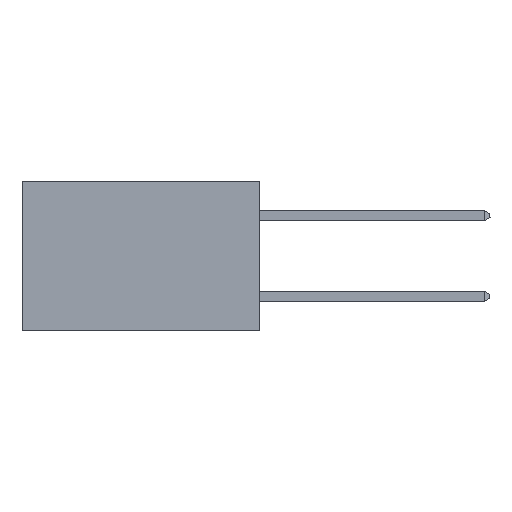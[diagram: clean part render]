
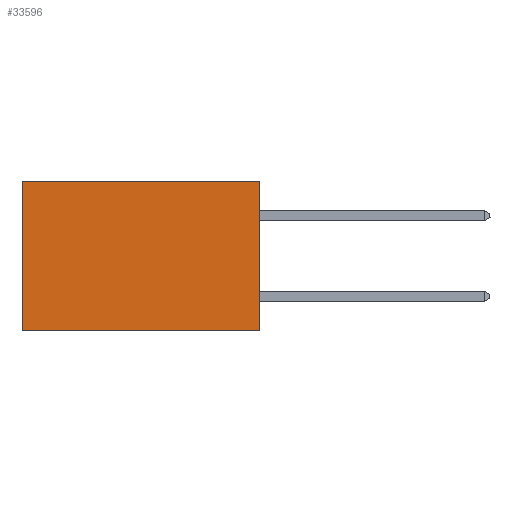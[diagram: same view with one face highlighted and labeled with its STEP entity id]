
A CAD part, left-side view. The second image highlights one B-rep face of the part: STEP entity #33596.
In plain terms, the highlighted planar face has unit normal (-1, 0, 0).
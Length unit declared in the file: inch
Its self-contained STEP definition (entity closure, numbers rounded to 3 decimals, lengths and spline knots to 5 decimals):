
#4 = DIRECTION ( 'NONE',  ( 0., 1., 0. ) ) ;
#1314 = DIRECTION ( 'NONE',  ( 0., 0., -1. ) ) ;
#4015 = DIRECTION ( 'NONE',  ( 0., 0., -1. ) ) ;
#4502 = CARTESIAN_POINT ( 'NONE',  ( 0.277, 0., -0.37 ) ) ;
#4627 = ORIENTED_EDGE ( 'NONE', *, *, #21180, .F. ) ;
#5019 = PLANE ( 'NONE',  #28074 ) ;
#5331 = VECTOR ( 'NONE', #12905, 39.37008 ) ;
#6145 = LINE ( 'NONE', #25647, #19620 ) ;
#6355 = VERTEX_POINT ( 'NONE', #24913 ) ;
#7911 = LINE ( 'NONE', #31600, #5331 ) ;
#8884 = EDGE_CURVE ( 'NONE', #18755, #31376, #24477, .T. ) ;
#9030 = ORIENTED_EDGE ( 'NONE', *, *, #8884, .F. ) ;
#10005 = VECTOR ( 'NONE', #4015, 39.37008 ) ;
#10516 = DIRECTION ( 'NONE',  ( 0., 0., -1. ) ) ;
#11281 = EDGE_CURVE ( 'NONE', #13461, #6355, #7911, .T. ) ;
#11825 = ORIENTED_EDGE ( 'NONE', *, *, #11281, .T. ) ;
#12905 = DIRECTION ( 'NONE',  ( 0., 1., 0. ) ) ;
#13461 = VERTEX_POINT ( 'NONE', #21602 ) ;
#16490 = VECTOR ( 'NONE', #4, 39.37008 ) ;
#18755 = VERTEX_POINT ( 'NONE', #4502 ) ;
#19620 = VECTOR ( 'NONE', #1314, 39.37008 ) ;
#21180 = EDGE_CURVE ( 'NONE', #13461, #18755, #30499, .T. ) ;
#21602 = CARTESIAN_POINT ( 'NONE',  ( 0.277, 0., 0. ) ) ;
#22875 = CARTESIAN_POINT ( 'NONE',  ( 0.277, 0., -0.37 ) ) ;
#23853 = CARTESIAN_POINT ( 'NONE',  ( 0.277, 0., -0.37 ) ) ;
#24405 = CARTESIAN_POINT ( 'NONE',  ( 0.277, 0., -0.37 ) ) ;
#24477 = LINE ( 'NONE', #24405, #16490 ) ;
#24913 = CARTESIAN_POINT ( 'NONE',  ( 0.277, 0.59, 0. ) ) ;
#25175 = FACE_OUTER_BOUND ( 'NONE', #32769, .T. ) ;
#25647 = CARTESIAN_POINT ( 'NONE',  ( 0.277, 0.59, -0.37 ) ) ;
#26515 = DIRECTION ( 'NONE',  ( 1., 0., 0. ) ) ;
#28074 = AXIS2_PLACEMENT_3D ( 'NONE', #23853, #26515, #10516 ) ;
#28314 = ORIENTED_EDGE ( 'NONE', *, *, #34828, .T. ) ;
#29142 = CARTESIAN_POINT ( 'NONE',  ( 0.277, 0.59, -0.37 ) ) ;
#30499 = LINE ( 'NONE', #22875, #10005 ) ;
#31376 = VERTEX_POINT ( 'NONE', #29142 ) ;
#31600 = CARTESIAN_POINT ( 'NONE',  ( 0.277, 0., 0. ) ) ;
#32769 = EDGE_LOOP ( 'NONE', ( #28314, #9030, #4627, #11825 ) ) ;
#33596 = ADVANCED_FACE ( 'NONE', ( #25175 ), #5019, .F. ) ;
#34828 = EDGE_CURVE ( 'NONE', #6355, #31376, #6145, .T. ) ;
